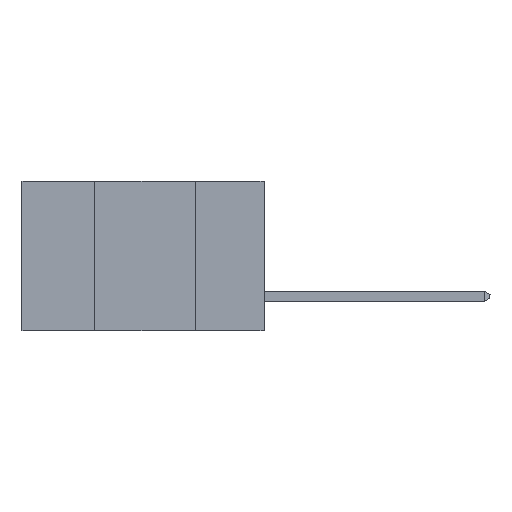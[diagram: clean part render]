
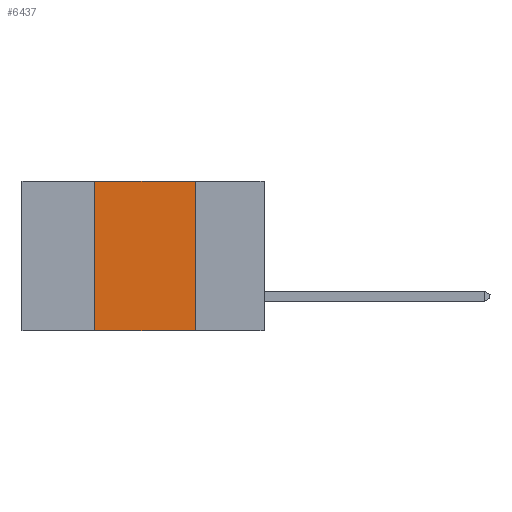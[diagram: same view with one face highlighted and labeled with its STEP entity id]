
A CAD part, left-side view. The second image highlights one B-rep face of the part: STEP entity #6437.
In plain terms, the highlighted planar face has unit normal (-1, 0, 0).
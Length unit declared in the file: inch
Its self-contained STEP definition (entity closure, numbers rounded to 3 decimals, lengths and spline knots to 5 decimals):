
#859 = VERTEX_POINT ( 'NONE', #9155 ) ;
#1057 = EDGE_CURVE ( 'NONE', #859, #21843, #5960, .T. ) ;
#1390 = CARTESIAN_POINT ( 'NONE',  ( 0., 0.17, -0.37 ) ) ;
#2054 = AXIS2_PLACEMENT_3D ( 'NONE', #17143, #16755, #24739 ) ;
#2064 = VERTEX_POINT ( 'NONE', #8373 ) ;
#2386 = VECTOR ( 'NONE', #16808, 39.37008 ) ;
#5713 = CARTESIAN_POINT ( 'NONE',  ( 0., 0.6, -0.37 ) ) ;
#5960 = LINE ( 'NONE', #5713, #24451 ) ;
#6437 = ADVANCED_FACE ( 'NONE', ( #8698 ), #13103, .F. ) ;
#7410 = VERTEX_POINT ( 'NONE', #11597 ) ;
#8130 = VECTOR ( 'NONE', #10614, 39.37008 ) ;
#8373 = CARTESIAN_POINT ( 'NONE',  ( 0., 0.17, 0. ) ) ;
#8698 = FACE_OUTER_BOUND ( 'NONE', #11765, .T. ) ;
#9155 = CARTESIAN_POINT ( 'NONE',  ( 0., 0.42, -0.37 ) ) ;
#10614 = DIRECTION ( 'NONE',  ( 0., 0., 1. ) ) ;
#11597 = CARTESIAN_POINT ( 'NONE',  ( 0., 0.42, 0. ) ) ;
#11761 = DIRECTION ( 'NONE',  ( 0., 0., -1. ) ) ;
#11765 = EDGE_LOOP ( 'NONE', ( #13241, #23912, #15105, #19767 ) ) ;
#12767 = CARTESIAN_POINT ( 'NONE',  ( 0., 0.6, 0. ) ) ;
#13103 = PLANE ( 'NONE',  #2054 ) ;
#13241 = ORIENTED_EDGE ( 'NONE', *, *, #18129, .F. ) ;
#13587 = LINE ( 'NONE', #18007, #24439 ) ;
#15105 = ORIENTED_EDGE ( 'NONE', *, *, #16592, .F. ) ;
#16354 = CARTESIAN_POINT ( 'NONE',  ( 0., 0.42, -0.37 ) ) ;
#16489 = LINE ( 'NONE', #16354, #8130 ) ;
#16592 = EDGE_CURVE ( 'NONE', #859, #7410, #16489, .T. ) ;
#16679 = LINE ( 'NONE', #12767, #2386 ) ;
#16755 = DIRECTION ( 'NONE',  ( 1., 0., 0. ) ) ;
#16808 = DIRECTION ( 'NONE',  ( 0., -1., 0. ) ) ;
#17143 = CARTESIAN_POINT ( 'NONE',  ( 0., 0.6, 0. ) ) ;
#18007 = CARTESIAN_POINT ( 'NONE',  ( 0., 0.17, -0.37 ) ) ;
#18129 = EDGE_CURVE ( 'NONE', #2064, #21843, #13587, .T. ) ;
#19767 = ORIENTED_EDGE ( 'NONE', *, *, #1057, .T. ) ;
#21617 = DIRECTION ( 'NONE',  ( 0., -1., 0. ) ) ;
#21675 = EDGE_CURVE ( 'NONE', #7410, #2064, #16679, .T. ) ;
#21843 = VERTEX_POINT ( 'NONE', #1390 ) ;
#23912 = ORIENTED_EDGE ( 'NONE', *, *, #21675, .F. ) ;
#24439 = VECTOR ( 'NONE', #11761, 39.37008 ) ;
#24451 = VECTOR ( 'NONE', #21617, 39.37008 ) ;
#24739 = DIRECTION ( 'NONE',  ( 0., 0., -1. ) ) ;
